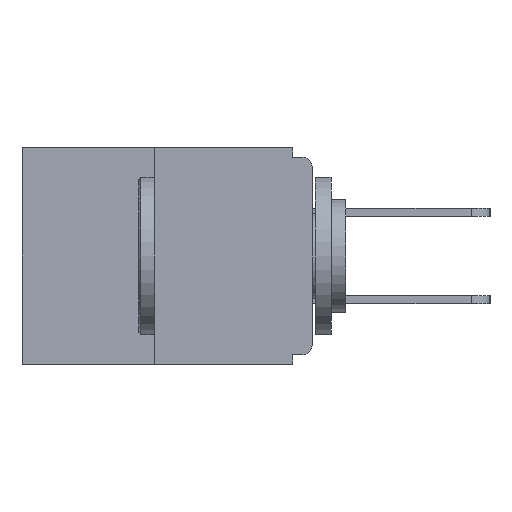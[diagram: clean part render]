
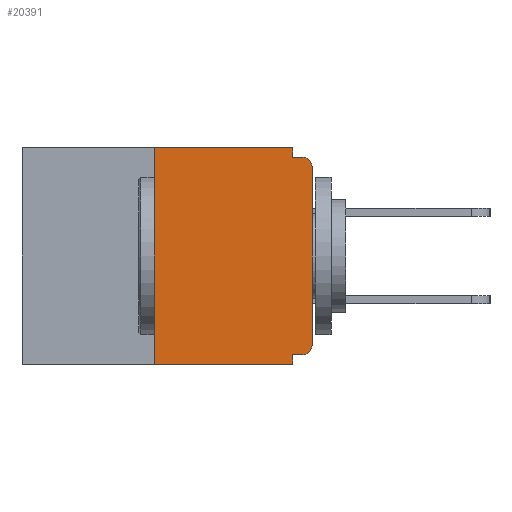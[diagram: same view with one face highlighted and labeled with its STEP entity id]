
A CAD part, left-side view. The second image highlights one B-rep face of the part: STEP entity #20391.
In plain terms, the highlighted planar face has unit normal (-1, 0, 0).
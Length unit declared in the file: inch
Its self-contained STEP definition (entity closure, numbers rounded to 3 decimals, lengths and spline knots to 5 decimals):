
#1133 = LINE ( 'NONE', #15513, #10424 ) ;
#1245 = VERTEX_POINT ( 'NONE', #5777 ) ;
#1450 = CARTESIAN_POINT ( 'NONE',  ( 0., 0.031, -0.015 ) ) ;
#1810 = VERTEX_POINT ( 'NONE', #25919 ) ;
#2042 = CARTESIAN_POINT ( 'NONE',  ( 0., 0.015, -0.328 ) ) ;
#2184 = ORIENTED_EDGE ( 'NONE', *, *, #24497, .F. ) ;
#3003 = CARTESIAN_POINT ( 'NONE',  ( 0., 0., -0.313 ) ) ;
#3275 = ORIENTED_EDGE ( 'NONE', *, *, #5704, .F. ) ;
#3448 = DIRECTION ( 'NONE',  ( 0., -1., 0. ) ) ;
#3485 = PLANE ( 'NONE',  #19782 ) ;
#3496 = ORIENTED_EDGE ( 'NONE', *, *, #3637, .T. ) ;
#3637 = EDGE_CURVE ( 'NONE', #18840, #9457, #25552, .T. ) ;
#4449 = ORIENTED_EDGE ( 'NONE', *, *, #4941, .F. ) ;
#4941 = EDGE_CURVE ( 'NONE', #22040, #25033, #20159, .T. ) ;
#5004 = VECTOR ( 'NONE', #8104, 39.37008 ) ;
#5378 = VECTOR ( 'NONE', #3448, 39.37008 ) ;
#5383 = VECTOR ( 'NONE', #7139, 39.37008 ) ;
#5704 = EDGE_CURVE ( 'NONE', #1245, #1810, #10466, .T. ) ;
#5777 = CARTESIAN_POINT ( 'NONE',  ( 0., 0.25, 0. ) ) ;
#5892 = CARTESIAN_POINT ( 'NONE',  ( 0., 0.031, -0.328 ) ) ;
#6430 = CARTESIAN_POINT ( 'NONE',  ( 0., 0., -0.03 ) ) ;
#6518 = ORIENTED_EDGE ( 'NONE', *, *, #11025, .T. ) ;
#7139 = DIRECTION ( 'NONE',  ( 0., -1., 0. ) ) ;
#7322 = CARTESIAN_POINT ( 'NONE',  ( 0., 0.46, -0.343 ) ) ;
#7633 = LINE ( 'NONE', #22820, #11933 ) ;
#8003 = CARTESIAN_POINT ( 'NONE',  ( 0., 0., -0.328 ) ) ;
#8104 = DIRECTION ( 'NONE',  ( 0., 1., 0. ) ) ;
#8126 = ORIENTED_EDGE ( 'NONE', *, *, #22544, .F. ) ;
#8560 = DIRECTION ( 'NONE',  ( -1., 0., 0. ) ) ;
#8729 = CARTESIAN_POINT ( 'NONE',  ( 0., 0.031, -0.343 ) ) ;
#9457 = VERTEX_POINT ( 'NONE', #14716 ) ;
#9472 = FACE_OUTER_BOUND ( 'NONE', #14976, .T. ) ;
#9537 = DIRECTION ( 'NONE',  ( 0., 0., -1. ) ) ;
#9790 = LINE ( 'NONE', #15571, #26935 ) ;
#10424 = VECTOR ( 'NONE', #11104, 39.37008 ) ;
#10462 = VERTEX_POINT ( 'NONE', #6430 ) ;
#10466 = LINE ( 'NONE', #17614, #20311 ) ;
#10877 = DIRECTION ( 'NONE',  ( 0., 0., 1. ) ) ;
#11025 = EDGE_CURVE ( 'NONE', #22040, #25691, #23080, .T. ) ;
#11104 = DIRECTION ( 'NONE',  ( 0., 0., -1. ) ) ;
#11181 = DIRECTION ( 'NONE',  ( 0., -1., 0. ) ) ;
#11603 = VECTOR ( 'NONE', #17199, 39.37008 ) ;
#11933 = VECTOR ( 'NONE', #10877, 39.37008 ) ;
#11950 = CARTESIAN_POINT ( 'NONE',  ( 0., 0., -0.015 ) ) ;
#12295 = ORIENTED_EDGE ( 'NONE', *, *, #16036, .T. ) ;
#13219 = CIRCLE ( 'NONE', #24133, 0.015 ) ;
#13293 = ORIENTED_EDGE ( 'NONE', *, *, #20826, .F. ) ;
#13798 = ORIENTED_EDGE ( 'NONE', *, *, #23993, .T. ) ;
#13931 = CARTESIAN_POINT ( 'NONE',  ( 0., 0.015, -0.03 ) ) ;
#14152 = AXIS2_PLACEMENT_3D ( 'NONE', #16782, #8560, #23112 ) ;
#14716 = CARTESIAN_POINT ( 'NONE',  ( 0., 0.031, -0.343 ) ) ;
#14976 = EDGE_LOOP ( 'NONE', ( #3275, #13293, #3496, #2184, #4449, #6518, #13798, #12295, #8126, #19274 ) ) ;
#15513 = CARTESIAN_POINT ( 'NONE',  ( 0., 0.031, 0. ) ) ;
#15571 = CARTESIAN_POINT ( 'NONE',  ( 0., 0.25, 0. ) ) ;
#16036 = EDGE_CURVE ( 'NONE', #10462, #25056, #13219, .T. ) ;
#16782 = CARTESIAN_POINT ( 'NONE',  ( 0., 0.015, -0.313 ) ) ;
#17199 = DIRECTION ( 'NONE',  ( 0., 0., -1. ) ) ;
#17614 = CARTESIAN_POINT ( 'NONE',  ( 0., 0.46, 0. ) ) ;
#18072 = CARTESIAN_POINT ( 'NONE',  ( 0., 0.46, 0. ) ) ;
#18840 = VERTEX_POINT ( 'NONE', #23318 ) ;
#19274 = ORIENTED_EDGE ( 'NONE', *, *, #21346, .F. ) ;
#19782 = AXIS2_PLACEMENT_3D ( 'NONE', #18072, #26745, #26654 ) ;
#19939 = DIRECTION ( 'NONE',  ( -1., 0., 0. ) ) ;
#20159 = LINE ( 'NONE', #8003, #5004 ) ;
#20311 = VECTOR ( 'NONE', #11181, 39.37008 ) ;
#20354 = VERTEX_POINT ( 'NONE', #1450 ) ;
#20364 = CARTESIAN_POINT ( 'NONE',  ( 0., 0.015, -0.015 ) ) ;
#20391 = ADVANCED_FACE ( 'NONE', ( #9472 ), #3485, .F. ) ;
#20473 = LINE ( 'NONE', #8729, #11603 ) ;
#20826 = EDGE_CURVE ( 'NONE', #18840, #1245, #9790, .T. ) ;
#21346 = EDGE_CURVE ( 'NONE', #1810, #20354, #1133, .T. ) ;
#21832 = DIRECTION ( 'NONE',  ( 0., 0., 1. ) ) ;
#22040 = VERTEX_POINT ( 'NONE', #2042 ) ;
#22544 = EDGE_CURVE ( 'NONE', #20354, #25056, #26509, .T. ) ;
#22820 = CARTESIAN_POINT ( 'NONE',  ( 0., 0., 0. ) ) ;
#23080 = CIRCLE ( 'NONE', #14152, 0.015 ) ;
#23112 = DIRECTION ( 'NONE',  ( 0., 0., -1. ) ) ;
#23318 = CARTESIAN_POINT ( 'NONE',  ( 0., 0.25, -0.343 ) ) ;
#23993 = EDGE_CURVE ( 'NONE', #25691, #10462, #7633, .T. ) ;
#24133 = AXIS2_PLACEMENT_3D ( 'NONE', #13931, #19939, #9537 ) ;
#24497 = EDGE_CURVE ( 'NONE', #25033, #9457, #20473, .T. ) ;
#25033 = VERTEX_POINT ( 'NONE', #5892 ) ;
#25056 = VERTEX_POINT ( 'NONE', #20364 ) ;
#25552 = LINE ( 'NONE', #7322, #5383 ) ;
#25691 = VERTEX_POINT ( 'NONE', #3003 ) ;
#25919 = CARTESIAN_POINT ( 'NONE',  ( 0., 0.031, 0. ) ) ;
#26509 = LINE ( 'NONE', #11950, #5378 ) ;
#26654 = DIRECTION ( 'NONE',  ( 0., 0., -1. ) ) ;
#26745 = DIRECTION ( 'NONE',  ( 1., 0., 0. ) ) ;
#26935 = VECTOR ( 'NONE', #21832, 39.37008 ) ;
